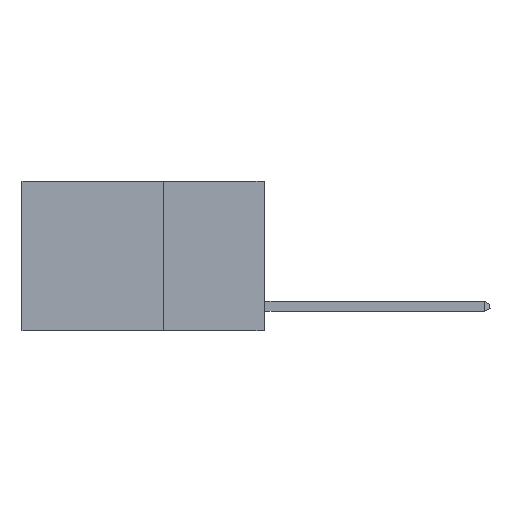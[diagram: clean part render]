
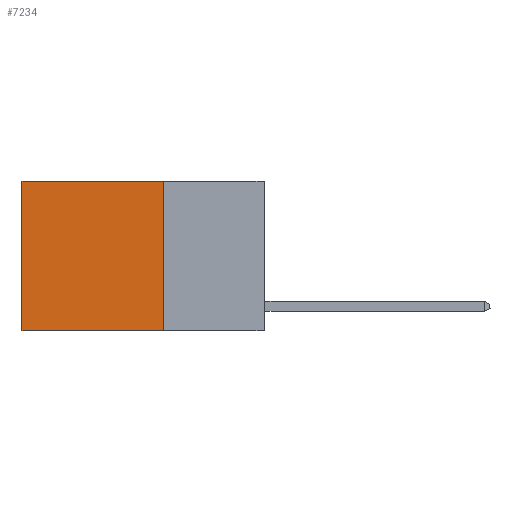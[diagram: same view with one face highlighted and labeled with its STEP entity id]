
A CAD part, left-side view. The second image highlights one B-rep face of the part: STEP entity #7234.
In plain terms, the highlighted planar face has unit normal (-1, 0, 0).
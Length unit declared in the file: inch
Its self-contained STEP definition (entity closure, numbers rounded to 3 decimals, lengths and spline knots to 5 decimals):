
#126 = DIRECTION ( 'NONE',  ( 0., 0., -1. ) ) ;
#771 = EDGE_CURVE ( 'NONE', #26017, #16493, #18602, .T. ) ;
#1611 = DIRECTION ( 'NONE',  ( 0., 1., 0. ) ) ;
#1702 = DIRECTION ( 'NONE',  ( 1., 0., 0. ) ) ;
#2272 = CARTESIAN_POINT ( 'NONE',  ( 0.2625, 0.6, 0. ) ) ;
#2834 = EDGE_CURVE ( 'NONE', #16493, #10194, #27946, .T. ) ;
#4813 = DIRECTION ( 'NONE',  ( 0., 1., 0. ) ) ;
#7234 = ADVANCED_FACE ( 'NONE', ( #16364 ), #12461, .F. ) ;
#9058 = CARTESIAN_POINT ( 'NONE',  ( 0.2625, 0.25, -0.37 ) ) ;
#9119 = LINE ( 'NONE', #15181, #14231 ) ;
#10194 = VERTEX_POINT ( 'NONE', #25175 ) ;
#11358 = VECTOR ( 'NONE', #1611, 39.37008 ) ;
#12054 = EDGE_CURVE ( 'NONE', #26120, #10194, #27297, .T. ) ;
#12461 = PLANE ( 'NONE',  #14303 ) ;
#14231 = VECTOR ( 'NONE', #126, 39.37008 ) ;
#14303 = AXIS2_PLACEMENT_3D ( 'NONE', #27622, #1702, #16816 ) ;
#15025 = ORIENTED_EDGE ( 'NONE', *, *, #12054, .F. ) ;
#15075 = VECTOR ( 'NONE', #17299, 39.37008 ) ;
#15181 = CARTESIAN_POINT ( 'NONE',  ( 0.2625, 0.25, 0. ) ) ;
#15617 = CARTESIAN_POINT ( 'NONE',  ( 0.2625, 0.25, 0. ) ) ;
#16329 = EDGE_CURVE ( 'NONE', #26017, #26120, #9119, .T. ) ;
#16364 = FACE_OUTER_BOUND ( 'NONE', #17255, .T. ) ;
#16493 = VERTEX_POINT ( 'NONE', #24559 ) ;
#16509 = ORIENTED_EDGE ( 'NONE', *, *, #2834, .T. ) ;
#16816 = DIRECTION ( 'NONE',  ( 0., 0., -1. ) ) ;
#17255 = EDGE_LOOP ( 'NONE', ( #16509, #15025, #22270, #23073 ) ) ;
#17299 = DIRECTION ( 'NONE',  ( 0., 0., -1. ) ) ;
#18602 = LINE ( 'NONE', #15617, #23685 ) ;
#21694 = CARTESIAN_POINT ( 'NONE',  ( 0.2625, 0.25, 0. ) ) ;
#22270 = ORIENTED_EDGE ( 'NONE', *, *, #16329, .F. ) ;
#23073 = ORIENTED_EDGE ( 'NONE', *, *, #771, .T. ) ;
#23685 = VECTOR ( 'NONE', #4813, 39.37008 ) ;
#24559 = CARTESIAN_POINT ( 'NONE',  ( 0.2625, 0.6, 0. ) ) ;
#25175 = CARTESIAN_POINT ( 'NONE',  ( 0.2625, 0.6, -0.37 ) ) ;
#26017 = VERTEX_POINT ( 'NONE', #21694 ) ;
#26120 = VERTEX_POINT ( 'NONE', #9058 ) ;
#27297 = LINE ( 'NONE', #27529, #11358 ) ;
#27529 = CARTESIAN_POINT ( 'NONE',  ( 0.2625, 0.25, -0.37 ) ) ;
#27622 = CARTESIAN_POINT ( 'NONE',  ( 0.2625, 0.25, 0. ) ) ;
#27946 = LINE ( 'NONE', #2272, #15075 ) ;
